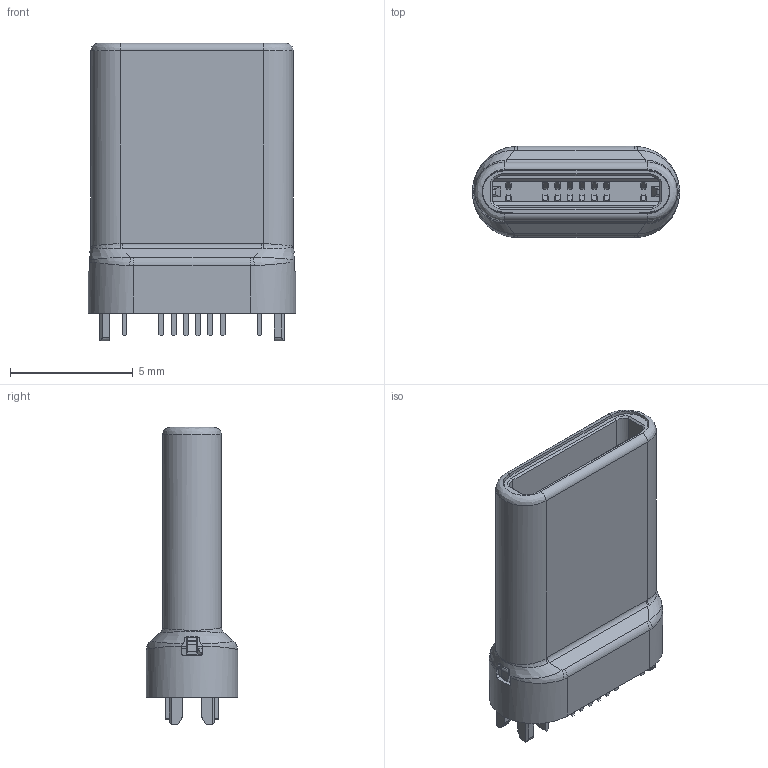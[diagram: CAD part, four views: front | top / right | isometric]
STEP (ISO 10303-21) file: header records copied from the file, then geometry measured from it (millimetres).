
FILE_DESCRIPTION (( 'STEP AP214' ), '1' );
FILE_NAME ('699B116-1A6-110.STEP', '2021-01-19T17:08:52', ( '' ), ( '' ), 'SwSTEP 2.0', 'SolidWorks 2020', '' );
FILE_SCHEMA (( 'AUTOMOTIVE_DESIGN' ));
Length unit declared in the file: millimetre
Products named in the file (4): Shell 699B116-1A6-11X; 699B116-1A6-110; Contacts 699B116-1A6-11X; Insulator 699B116-1A6-11X_White
Assembly tree (3 placements, depth 2):
  699B116-1A6-110
    Contacts 699B116-1A6-11X
    Insulator 699B116-1A6-11X_White
    Shell 699B116-1A6-11X
Bounding box: 8.45 x 3.72 x 12.13 mm (x, y, z)
Volume: 171.1 mm3; surface area: 1247.7 mm2
Topology: 19 solids, 19 shells, 1586 faces, 4573 edges, 2985 vertices
Faces by surface type: plane 985, cylinder 498, bspline 64, cone 39
Entity records: 55870 total; most frequent: CARTESIAN_POINT 14419, ORIENTED_EDGE 9142, DIRECTION 8081, EDGE_CURVE 4571, VECTOR 3173, LINE 3173, VERTEX_POINT 2985, AXIS2_PLACEMENT_3D 2454
